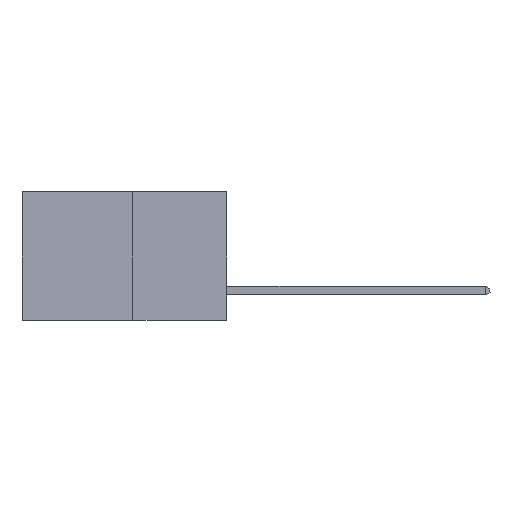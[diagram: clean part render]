
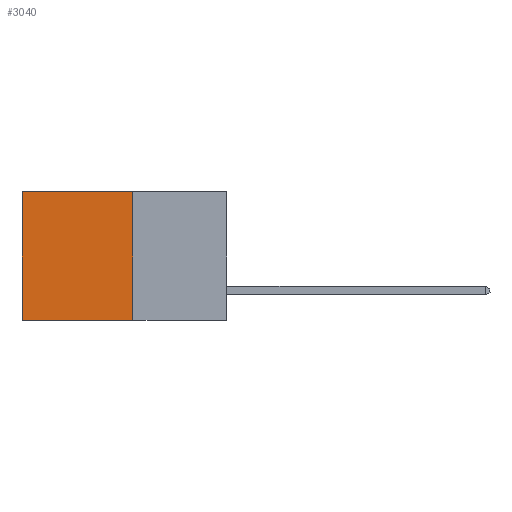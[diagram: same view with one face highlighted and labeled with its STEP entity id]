
A CAD part, left-side view. The second image highlights one B-rep face of the part: STEP entity #3040.
In plain terms, the highlighted planar face has unit normal (-1, 0, 0).
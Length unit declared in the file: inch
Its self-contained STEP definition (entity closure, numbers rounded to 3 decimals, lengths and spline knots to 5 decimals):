
#980 = FACE_OUTER_BOUND ( 'NONE', #25359, .T. ) ;
#2497 = EDGE_CURVE ( 'NONE', #24806, #3685, #3915, .T. ) ;
#2870 = CARTESIAN_POINT ( 'NONE',  ( 0.277, 0.27, 0. ) ) ;
#2927 = ORIENTED_EDGE ( 'NONE', *, *, #27513, .F. ) ;
#3040 = ADVANCED_FACE ( 'NONE', ( #980 ), #4104, .F. ) ;
#3685 = VERTEX_POINT ( 'NONE', #16242 ) ;
#3915 = LINE ( 'NONE', #17261, #21863 ) ;
#3998 = DIRECTION ( 'NONE',  ( 0., 0., -1. ) ) ;
#4040 = DIRECTION ( 'NONE',  ( 1., 0., 0. ) ) ;
#4071 = CARTESIAN_POINT ( 'NONE',  ( 0.277, 0.27, -0.37 ) ) ;
#4104 = PLANE ( 'NONE',  #7549 ) ;
#7524 = DIRECTION ( 'NONE',  ( 0., 1., 0. ) ) ;
#7549 = AXIS2_PLACEMENT_3D ( 'NONE', #4071, #4040, #3998 ) ;
#9375 = DIRECTION ( 'NONE',  ( 0., 0., -1. ) ) ;
#10552 = VERTEX_POINT ( 'NONE', #11387 ) ;
#11387 = CARTESIAN_POINT ( 'NONE',  ( 0.277, 0.27, -0.37 ) ) ;
#12754 = VECTOR ( 'NONE', #9375, 39.37008 ) ;
#13746 = CARTESIAN_POINT ( 'NONE',  ( 0.277, 0.27, -0.37 ) ) ;
#14453 = CARTESIAN_POINT ( 'NONE',  ( 0.277, 0.27, 0. ) ) ;
#15404 = ORIENTED_EDGE ( 'NONE', *, *, #2497, .T. ) ;
#16242 = CARTESIAN_POINT ( 'NONE',  ( 0.277, 0.59, -0.37 ) ) ;
#16280 = CARTESIAN_POINT ( 'NONE',  ( 0.277, 0.59, 0. ) ) ;
#17261 = CARTESIAN_POINT ( 'NONE',  ( 0.277, 0.59, -0.37 ) ) ;
#17354 = DIRECTION ( 'NONE',  ( 0., 0., -1. ) ) ;
#17641 = VECTOR ( 'NONE', #7524, 39.37008 ) ;
#17855 = VERTEX_POINT ( 'NONE', #14453 ) ;
#18755 = LINE ( 'NONE', #13746, #12754 ) ;
#19149 = ORIENTED_EDGE ( 'NONE', *, *, #24175, .T. ) ;
#20884 = EDGE_CURVE ( 'NONE', #10552, #3685, #23518, .T. ) ;
#21863 = VECTOR ( 'NONE', #17354, 39.37008 ) ;
#23044 = ORIENTED_EDGE ( 'NONE', *, *, #20884, .F. ) ;
#23099 = CARTESIAN_POINT ( 'NONE',  ( 0.277, 0.27, -0.37 ) ) ;
#23518 = LINE ( 'NONE', #23099, #17641 ) ;
#24175 = EDGE_CURVE ( 'NONE', #17855, #24806, #26848, .T. ) ;
#24806 = VERTEX_POINT ( 'NONE', #16280 ) ;
#25359 = EDGE_LOOP ( 'NONE', ( #15404, #23044, #2927, #19149 ) ) ;
#26151 = VECTOR ( 'NONE', #27393, 39.37008 ) ;
#26848 = LINE ( 'NONE', #2870, #26151 ) ;
#27393 = DIRECTION ( 'NONE',  ( 0., 1., 0. ) ) ;
#27513 = EDGE_CURVE ( 'NONE', #17855, #10552, #18755, .T. ) ;
